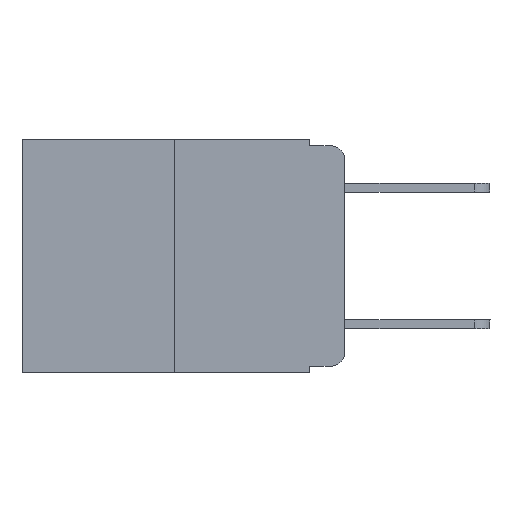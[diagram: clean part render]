
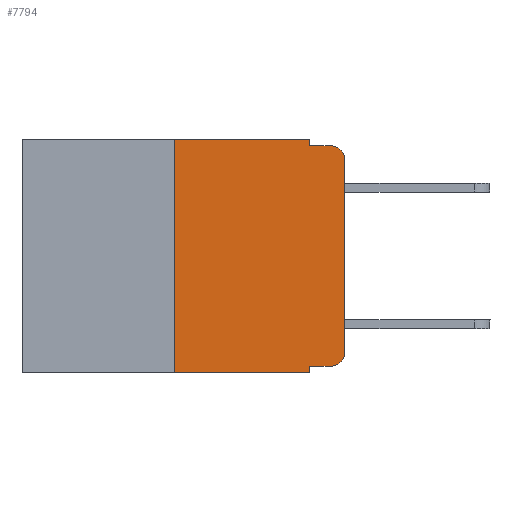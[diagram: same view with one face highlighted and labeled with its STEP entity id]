
A CAD part, left-side view. The second image highlights one B-rep face of the part: STEP entity #7794.
In plain terms, the highlighted planar face has unit normal (-1, 0, 0).
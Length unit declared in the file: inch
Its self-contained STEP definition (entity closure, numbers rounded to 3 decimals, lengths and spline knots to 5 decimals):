
#7 = LINE ( 'NONE', #14434, #10043 ) ;
#164 = CARTESIAN_POINT ( 'NONE',  ( 0., 0.051, 0. ) ) ;
#752 = VERTEX_POINT ( 'NONE', #18705 ) ;
#860 = DIRECTION ( 'NONE',  ( 0., -1., 0. ) ) ;
#959 = LINE ( 'NONE', #15510, #18782 ) ;
#1067 = ORIENTED_EDGE ( 'NONE', *, *, #4868, .T. ) ;
#1169 = LINE ( 'NONE', #16191, #20256 ) ;
#1210 = EDGE_CURVE ( 'NONE', #2782, #1572, #3935, .T. ) ;
#1391 = CARTESIAN_POINT ( 'NONE',  ( 0., 0.473, 0. ) ) ;
#1457 = DIRECTION ( 'NONE',  ( 0., 0., -1. ) ) ;
#1572 = VERTEX_POINT ( 'NONE', #9759 ) ;
#1816 = VECTOR ( 'NONE', #14720, 39.37008 ) ;
#1826 = DIRECTION ( 'NONE',  ( 0., 0., -1. ) ) ;
#2062 = LINE ( 'NONE', #10036, #1816 ) ;
#2273 = EDGE_CURVE ( 'NONE', #15508, #752, #10051, .T. ) ;
#2525 = EDGE_CURVE ( 'NONE', #752, #12767, #959, .T. ) ;
#2782 = VERTEX_POINT ( 'NONE', #19545 ) ;
#2862 = AXIS2_PLACEMENT_3D ( 'NONE', #15641, #16975, #13908 ) ;
#3344 = LINE ( 'NONE', #9481, #3606 ) ;
#3606 = VECTOR ( 'NONE', #8179, 39.37008 ) ;
#3704 = ORIENTED_EDGE ( 'NONE', *, *, #1210, .F. ) ;
#3935 = LINE ( 'NONE', #8885, #5151 ) ;
#3968 = EDGE_CURVE ( 'NONE', #4130, #15220, #3344, .T. ) ;
#4052 = ORIENTED_EDGE ( 'NONE', *, *, #13769, .F. ) ;
#4130 = VERTEX_POINT ( 'NONE', #11962 ) ;
#4301 = VECTOR ( 'NONE', #860, 39.37008 ) ;
#4358 = CARTESIAN_POINT ( 'NONE',  ( 0., 0.051, -0.01 ) ) ;
#4484 = EDGE_CURVE ( 'NONE', #12767, #12668, #16452, .T. ) ;
#4715 = EDGE_LOOP ( 'NONE', ( #16686, #8693, #4052, #4859, #20083, #19004, #7680, #3704, #1067, #6725 ) ) ;
#4721 = EDGE_CURVE ( 'NONE', #15220, #10457, #2062, .T. ) ;
#4859 = ORIENTED_EDGE ( 'NONE', *, *, #4721, .F. ) ;
#4868 = EDGE_CURVE ( 'NONE', #2782, #15508, #5279, .T. ) ;
#5151 = VECTOR ( 'NONE', #18236, 39.37008 ) ;
#5279 = LINE ( 'NONE', #8666, #4301 ) ;
#5351 = CARTESIAN_POINT ( 'NONE',  ( 0., 0.02, -0.333 ) ) ;
#6716 = DIRECTION ( 'NONE',  ( -1., 0., 0. ) ) ;
#6725 = ORIENTED_EDGE ( 'NONE', *, *, #2273, .T. ) ;
#6895 = EDGE_CURVE ( 'NONE', #19728, #1572, #7, .T. ) ;
#7459 = AXIS2_PLACEMENT_3D ( 'NONE', #1391, #20452, #1457 ) ;
#7486 = DIRECTION ( 'NONE',  ( 0., -1., 0. ) ) ;
#7680 = ORIENTED_EDGE ( 'NONE', *, *, #6895, .T. ) ;
#7794 = ADVANCED_FACE ( 'NONE', ( #15505 ), #7867, .F. ) ;
#7822 = CARTESIAN_POINT ( 'NONE',  ( 0., 0.02, -0.01 ) ) ;
#7852 = EDGE_CURVE ( 'NONE', #19728, #4130, #1169, .T. ) ;
#7867 = PLANE ( 'NONE',  #7459 ) ;
#8114 = DIRECTION ( 'NONE',  ( 0., -1., 0. ) ) ;
#8179 = DIRECTION ( 'NONE',  ( 0., -1., 0. ) ) ;
#8666 = CARTESIAN_POINT ( 'NONE',  ( 0., 0.051, -0.333 ) ) ;
#8693 = ORIENTED_EDGE ( 'NONE', *, *, #4484, .T. ) ;
#8885 = CARTESIAN_POINT ( 'NONE',  ( 0., 0.051, 0. ) ) ;
#9168 = DIRECTION ( 'NONE',  ( 0., 0., 1. ) ) ;
#9481 = CARTESIAN_POINT ( 'NONE',  ( 0., 0.473, 0. ) ) ;
#9759 = CARTESIAN_POINT ( 'NONE',  ( 0., 0.051, -0.343 ) ) ;
#10036 = CARTESIAN_POINT ( 'NONE',  ( 0., 0.051, 0. ) ) ;
#10043 = VECTOR ( 'NONE', #8114, 39.37008 ) ;
#10051 = CIRCLE ( 'NONE', #20212, 0.02 ) ;
#10457 = VERTEX_POINT ( 'NONE', #12846 ) ;
#10711 = CARTESIAN_POINT ( 'NONE',  ( 0., 0.25, -0.343 ) ) ;
#11962 = CARTESIAN_POINT ( 'NONE',  ( 0., 0.25, 0. ) ) ;
#12668 = VERTEX_POINT ( 'NONE', #7822 ) ;
#12767 = VERTEX_POINT ( 'NONE', #17401 ) ;
#12846 = CARTESIAN_POINT ( 'NONE',  ( 0., 0.051, -0.01 ) ) ;
#13026 = CARTESIAN_POINT ( 'NONE',  ( 0., 0.02, -0.313 ) ) ;
#13769 = EDGE_CURVE ( 'NONE', #10457, #12668, #19204, .T. ) ;
#13908 = DIRECTION ( 'NONE',  ( 0., 0., -1. ) ) ;
#14434 = CARTESIAN_POINT ( 'NONE',  ( 0., 0.473, -0.343 ) ) ;
#14720 = DIRECTION ( 'NONE',  ( 0., 0., -1. ) ) ;
#15220 = VERTEX_POINT ( 'NONE', #164 ) ;
#15505 = FACE_OUTER_BOUND ( 'NONE', #4715, .T. ) ;
#15508 = VERTEX_POINT ( 'NONE', #5351 ) ;
#15510 = CARTESIAN_POINT ( 'NONE',  ( 0., 0., 0. ) ) ;
#15641 = CARTESIAN_POINT ( 'NONE',  ( 0., 0.02, -0.03 ) ) ;
#16049 = DIRECTION ( 'NONE',  ( 0., 0., 1. ) ) ;
#16191 = CARTESIAN_POINT ( 'NONE',  ( 0., 0.25, 0. ) ) ;
#16452 = CIRCLE ( 'NONE', #2862, 0.02 ) ;
#16686 = ORIENTED_EDGE ( 'NONE', *, *, #2525, .T. ) ;
#16975 = DIRECTION ( 'NONE',  ( -1., 0., 0. ) ) ;
#17401 = CARTESIAN_POINT ( 'NONE',  ( 0., 0., -0.03 ) ) ;
#18236 = DIRECTION ( 'NONE',  ( 0., 0., -1. ) ) ;
#18705 = CARTESIAN_POINT ( 'NONE',  ( 0., 0., -0.313 ) ) ;
#18782 = VECTOR ( 'NONE', #9168, 39.37008 ) ;
#19004 = ORIENTED_EDGE ( 'NONE', *, *, #7852, .F. ) ;
#19204 = LINE ( 'NONE', #4358, #20443 ) ;
#19545 = CARTESIAN_POINT ( 'NONE',  ( 0., 0.051, -0.333 ) ) ;
#19728 = VERTEX_POINT ( 'NONE', #10711 ) ;
#20083 = ORIENTED_EDGE ( 'NONE', *, *, #3968, .F. ) ;
#20212 = AXIS2_PLACEMENT_3D ( 'NONE', #13026, #6716, #1826 ) ;
#20256 = VECTOR ( 'NONE', #16049, 39.37008 ) ;
#20443 = VECTOR ( 'NONE', #7486, 39.37008 ) ;
#20452 = DIRECTION ( 'NONE',  ( 1., 0., 0. ) ) ;
